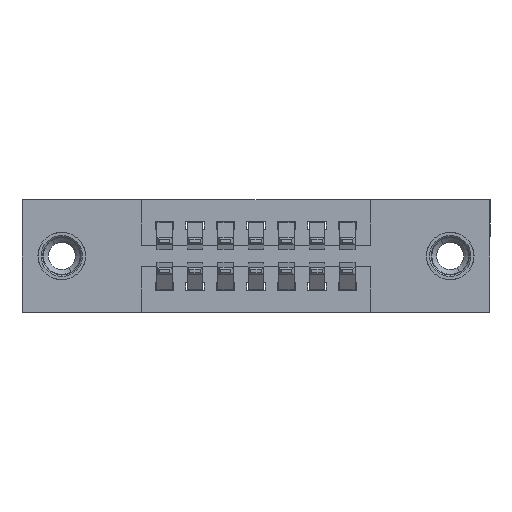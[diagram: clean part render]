
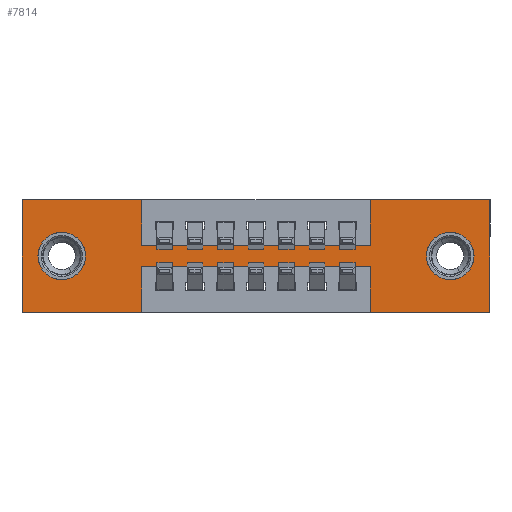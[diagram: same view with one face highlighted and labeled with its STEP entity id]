
A CAD part, front view. The second image highlights one B-rep face of the part: STEP entity #7814.
In plain terms, the highlighted planar face has unit normal (0, -1, 0).
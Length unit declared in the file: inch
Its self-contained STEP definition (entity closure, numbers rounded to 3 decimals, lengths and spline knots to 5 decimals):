
#158 = AXIS2_PLACEMENT_3D ( 'NONE', #3073, #11165, #8656 ) ;
#257 = LINE ( 'NONE', #6389, #11113 ) ;
#455 = CARTESIAN_POINT ( 'NONE',  ( 1.405, 0., -0.185 ) ) ;
#667 = CARTESIAN_POINT ( 'NONE',  ( 1.1425, 0., -0.37 ) ) ;
#693 = CARTESIAN_POINT ( 'NONE',  ( 0.3925, 0., 0. ) ) ;
#1232 = AXIS2_PLACEMENT_3D ( 'NONE', #455, #11784, #1466 ) ;
#1240 = EDGE_LOOP ( 'NONE', ( #9123, #6978, #14030, #5935, #3427, #2451, #12531, #4812, #10396, #8191, #2768, #3235 ) ) ;
#1307 = LINE ( 'NONE', #8569, #6029 ) ;
#1466 = DIRECTION ( 'NONE',  ( 0., 0., -1. ) ) ;
#1530 = EDGE_CURVE ( 'NONE', #7861, #12198, #13733, .T. ) ;
#1538 = VECTOR ( 'NONE', #9657, 39.37008 ) ;
#1640 = DIRECTION ( 'NONE',  ( -1., 0., 0. ) ) ;
#1662 = VERTEX_POINT ( 'NONE', #4846 ) ;
#1707 = LINE ( 'NONE', #14265, #7528 ) ;
#1783 = AXIS2_PLACEMENT_3D ( 'NONE', #11985, #2997, #4732 ) ;
#1846 = DIRECTION ( 'NONE',  ( 0., -1., 0. ) ) ;
#1911 = DIRECTION ( 'NONE',  ( 0., 0., -1. ) ) ;
#1941 = CARTESIAN_POINT ( 'NONE',  ( 0., 0., 0. ) ) ;
#1994 = DIRECTION ( 'NONE',  ( 1., 0., 0. ) ) ;
#2135 = AXIS2_PLACEMENT_3D ( 'NONE', #7586, #1846, #9960 ) ;
#2391 = LINE ( 'NONE', #12134, #11471 ) ;
#2451 = ORIENTED_EDGE ( 'NONE', *, *, #5394, .F. ) ;
#2527 = VECTOR ( 'NONE', #1994, 39.37008 ) ;
#2531 = VERTEX_POINT ( 'NONE', #5413 ) ;
#2690 = DIRECTION ( 'NONE',  ( 0., 0., 1. ) ) ;
#2762 = EDGE_CURVE ( 'NONE', #3521, #7861, #5989, .T. ) ;
#2768 = ORIENTED_EDGE ( 'NONE', *, *, #12354, .F. ) ;
#2783 = CIRCLE ( 'NONE', #158, 0.078 ) ;
#2824 = DIRECTION ( 'NONE',  ( 0., 0., -1. ) ) ;
#2997 = DIRECTION ( 'NONE',  ( 0., 1., 0. ) ) ;
#3019 = LINE ( 'NONE', #7782, #10847 ) ;
#3073 = CARTESIAN_POINT ( 'NONE',  ( 0.13, 0., -0.185 ) ) ;
#3233 = DIRECTION ( 'NONE',  ( 0., 1., 0. ) ) ;
#3235 = ORIENTED_EDGE ( 'NONE', *, *, #12171, .F. ) ;
#3271 = VECTOR ( 'NONE', #2690, 39.37008 ) ;
#3427 = ORIENTED_EDGE ( 'NONE', *, *, #14055, .F. ) ;
#3521 = VERTEX_POINT ( 'NONE', #11852 ) ;
#3875 = VECTOR ( 'NONE', #8976, 39.37008 ) ;
#3902 = DIRECTION ( 'NONE',  ( 0., 0., -1. ) ) ;
#4104 = VERTEX_POINT ( 'NONE', #6522 ) ;
#4354 = CARTESIAN_POINT ( 'NONE',  ( 1.1425, 0., -0.15 ) ) ;
#4423 = VECTOR ( 'NONE', #4561, 39.37008 ) ;
#4554 = FACE_BOUND ( 'NONE', #13389, .T. ) ;
#4561 = DIRECTION ( 'NONE',  ( -1., 0., 0. ) ) ;
#4618 = EDGE_LOOP ( 'NONE', ( #8648, #5249 ) ) ;
#4732 = DIRECTION ( 'NONE',  ( 0., 0., 1. ) ) ;
#4812 = ORIENTED_EDGE ( 'NONE', *, *, #2762, .F. ) ;
#4846 = CARTESIAN_POINT ( 'NONE',  ( 0., 0., -0.37 ) ) ;
#4913 = VERTEX_POINT ( 'NONE', #7428 ) ;
#5249 = ORIENTED_EDGE ( 'NONE', *, *, #12593, .T. ) ;
#5394 = EDGE_CURVE ( 'NONE', #12198, #10551, #10608, .T. ) ;
#5413 = CARTESIAN_POINT ( 'NONE',  ( 1.1425, 0., -0.22 ) ) ;
#5437 = CARTESIAN_POINT ( 'NONE',  ( 0.3925, 0., -0.15 ) ) ;
#5923 = VERTEX_POINT ( 'NONE', #11648 ) ;
#5935 = ORIENTED_EDGE ( 'NONE', *, *, #13168, .F. ) ;
#5989 = LINE ( 'NONE', #5437, #2527 ) ;
#6029 = VECTOR ( 'NONE', #1640, 39.37008 ) ;
#6102 = EDGE_CURVE ( 'NONE', #6816, #9800, #12984, .T. ) ;
#6246 = VERTEX_POINT ( 'NONE', #12113 ) ;
#6389 = CARTESIAN_POINT ( 'NONE',  ( 1.535, 0., 0. ) ) ;
#6491 = ORIENTED_EDGE ( 'NONE', *, *, #14313, .T. ) ;
#6522 = CARTESIAN_POINT ( 'NONE',  ( 0.13, 0., -0.107 ) ) ;
#6676 = CARTESIAN_POINT ( 'NONE',  ( 1.405, 0., -0.185 ) ) ;
#6816 = VERTEX_POINT ( 'NONE', #7863 ) ;
#6953 = CARTESIAN_POINT ( 'NONE',  ( 0., 0., 0. ) ) ;
#6978 = ORIENTED_EDGE ( 'NONE', *, *, #13976, .F. ) ;
#7400 = VERTEX_POINT ( 'NONE', #6953 ) ;
#7428 = CARTESIAN_POINT ( 'NONE',  ( 0.13, 0., -0.263 ) ) ;
#7443 = CARTESIAN_POINT ( 'NONE',  ( 0., 0., 0. ) ) ;
#7528 = VECTOR ( 'NONE', #9468, 39.37008 ) ;
#7586 = CARTESIAN_POINT ( 'NONE',  ( 0., 0., -0.37 ) ) ;
#7782 = CARTESIAN_POINT ( 'NONE',  ( 0.3925, 0., -0.37 ) ) ;
#7814 = ADVANCED_FACE ( 'NONE', ( #14283, #4554, #13553 ), #11089, .T. ) ;
#7861 = VERTEX_POINT ( 'NONE', #4354 ) ;
#7863 = CARTESIAN_POINT ( 'NONE',  ( 1.405, 0., -0.107 ) ) ;
#8012 = CARTESIAN_POINT ( 'NONE',  ( 0.3925, 0., -0.22 ) ) ;
#8191 = ORIENTED_EDGE ( 'NONE', *, *, #8817, .F. ) ;
#8213 = CIRCLE ( 'NONE', #11593, 0.078 ) ;
#8216 = EDGE_CURVE ( 'NONE', #6246, #3521, #13890, .T. ) ;
#8421 = CARTESIAN_POINT ( 'NONE',  ( 0., 0., 0. ) ) ;
#8569 = CARTESIAN_POINT ( 'NONE',  ( 0.3925, 0., -0.22 ) ) ;
#8648 = ORIENTED_EDGE ( 'NONE', *, *, #6102, .T. ) ;
#8656 = DIRECTION ( 'NONE',  ( 0., 0., 1. ) ) ;
#8817 = EDGE_CURVE ( 'NONE', #7400, #6246, #10356, .T. ) ;
#8976 = DIRECTION ( 'NONE',  ( 1., 0., 0. ) ) ;
#9123 = ORIENTED_EDGE ( 'NONE', *, *, #10849, .F. ) ;
#9461 = VECTOR ( 'NONE', #2824, 39.37008 ) ;
#9468 = DIRECTION ( 'NONE',  ( -1., 0., 0. ) ) ;
#9649 = CIRCLE ( 'NONE', #1783, 0.078 ) ;
#9657 = DIRECTION ( 'NONE',  ( 0., 0., 1. ) ) ;
#9800 = VERTEX_POINT ( 'NONE', #13148 ) ;
#9960 = DIRECTION ( 'NONE',  ( 0., 0., -1. ) ) ;
#10356 = LINE ( 'NONE', #7443, #14776 ) ;
#10396 = ORIENTED_EDGE ( 'NONE', *, *, #8216, .F. ) ;
#10551 = VERTEX_POINT ( 'NONE', #12018 ) ;
#10608 = LINE ( 'NONE', #1941, #3875 ) ;
#10662 = CARTESIAN_POINT ( 'NONE',  ( 1.1425, 0., 0. ) ) ;
#10847 = VECTOR ( 'NONE', #1911, 39.37008 ) ;
#10849 = EDGE_CURVE ( 'NONE', #12196, #5923, #3019, .T. ) ;
#10895 = DIRECTION ( 'NONE',  ( 0., 0., 1. ) ) ;
#11089 = PLANE ( 'NONE',  #2135 ) ;
#11113 = VECTOR ( 'NONE', #3902, 39.37008 ) ;
#11165 = DIRECTION ( 'NONE',  ( 0., 1., 0. ) ) ;
#11471 = VECTOR ( 'NONE', #10895, 39.37008 ) ;
#11593 = AXIS2_PLACEMENT_3D ( 'NONE', #6676, #3233, #13745 ) ;
#11648 = CARTESIAN_POINT ( 'NONE',  ( 0.3925, 0., -0.37 ) ) ;
#11784 = DIRECTION ( 'NONE',  ( 0., 1., 0. ) ) ;
#11852 = CARTESIAN_POINT ( 'NONE',  ( 0.3925, 0., -0.15 ) ) ;
#11985 = CARTESIAN_POINT ( 'NONE',  ( 0.13, 0., -0.185 ) ) ;
#12018 = CARTESIAN_POINT ( 'NONE',  ( 1.535, 0., 0. ) ) ;
#12113 = CARTESIAN_POINT ( 'NONE',  ( 0.3925, 0., 0. ) ) ;
#12134 = CARTESIAN_POINT ( 'NONE',  ( 1.1425, 0., -0.37 ) ) ;
#12171 = EDGE_CURVE ( 'NONE', #5923, #1662, #12650, .T. ) ;
#12196 = VERTEX_POINT ( 'NONE', #8012 ) ;
#12198 = VERTEX_POINT ( 'NONE', #12686 ) ;
#12354 = EDGE_CURVE ( 'NONE', #1662, #7400, #13009, .T. ) ;
#12531 = ORIENTED_EDGE ( 'NONE', *, *, #1530, .F. ) ;
#12593 = EDGE_CURVE ( 'NONE', #9800, #6816, #8213, .T. ) ;
#12650 = LINE ( 'NONE', #13761, #4423 ) ;
#12686 = CARTESIAN_POINT ( 'NONE',  ( 1.1425, 0., 0. ) ) ;
#12965 = EDGE_CURVE ( 'NONE', #4913, #4104, #2783, .T. ) ;
#12984 = CIRCLE ( 'NONE', #1232, 0.078 ) ;
#13009 = LINE ( 'NONE', #8421, #1538 ) ;
#13148 = CARTESIAN_POINT ( 'NONE',  ( 1.405, 0., -0.263 ) ) ;
#13168 = EDGE_CURVE ( 'NONE', #13396, #14040, #1707, .T. ) ;
#13389 = EDGE_LOOP ( 'NONE', ( #6491, #14109 ) ) ;
#13396 = VERTEX_POINT ( 'NONE', #14652 ) ;
#13553 = FACE_OUTER_BOUND ( 'NONE', #1240, .T. ) ;
#13733 = LINE ( 'NONE', #10662, #3271 ) ;
#13745 = DIRECTION ( 'NONE',  ( 0., 0., -1. ) ) ;
#13761 = CARTESIAN_POINT ( 'NONE',  ( 0., 0., -0.37 ) ) ;
#13890 = LINE ( 'NONE', #693, #9461 ) ;
#13976 = EDGE_CURVE ( 'NONE', #2531, #12196, #1307, .T. ) ;
#14015 = EDGE_CURVE ( 'NONE', #14040, #2531, #2391, .T. ) ;
#14030 = ORIENTED_EDGE ( 'NONE', *, *, #14015, .F. ) ;
#14040 = VERTEX_POINT ( 'NONE', #667 ) ;
#14055 = EDGE_CURVE ( 'NONE', #10551, #13396, #257, .T. ) ;
#14109 = ORIENTED_EDGE ( 'NONE', *, *, #12965, .T. ) ;
#14265 = CARTESIAN_POINT ( 'NONE',  ( 0., 0., -0.37 ) ) ;
#14283 = FACE_BOUND ( 'NONE', #4618, .T. ) ;
#14313 = EDGE_CURVE ( 'NONE', #4104, #4913, #9649, .T. ) ;
#14357 = DIRECTION ( 'NONE',  ( 1., 0., 0. ) ) ;
#14652 = CARTESIAN_POINT ( 'NONE',  ( 1.535, 0., -0.37 ) ) ;
#14776 = VECTOR ( 'NONE', #14357, 39.37008 ) ;
